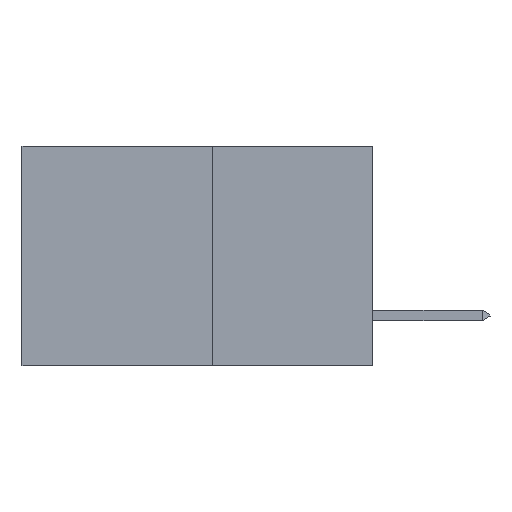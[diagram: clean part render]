
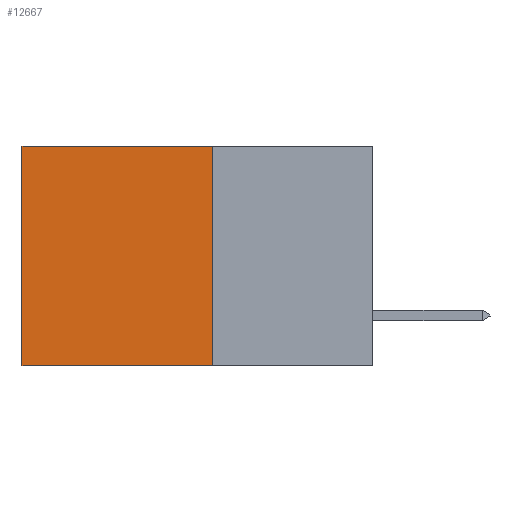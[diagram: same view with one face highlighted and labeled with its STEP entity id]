
A CAD part, left-side view. The second image highlights one B-rep face of the part: STEP entity #12667.
In plain terms, the highlighted planar face has unit normal (-1, 0, 0).
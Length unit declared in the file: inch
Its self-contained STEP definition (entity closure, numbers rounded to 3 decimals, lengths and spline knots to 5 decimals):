
#246 = CARTESIAN_POINT ( 'NONE',  ( 0.277, 0.27, -0.37 ) ) ;
#333 = DIRECTION ( 'NONE',  ( 0., 0., -1. ) ) ;
#2335 = VECTOR ( 'NONE', #3183, 39.37008 ) ;
#2690 = PLANE ( 'NONE',  #11968 ) ;
#3013 = DIRECTION ( 'NONE',  ( 0., 0., -1. ) ) ;
#3183 = DIRECTION ( 'NONE',  ( 0., 1., 0. ) ) ;
#4940 = VECTOR ( 'NONE', #3013, 39.37008 ) ;
#5059 = CARTESIAN_POINT ( 'NONE',  ( 0.277, 0.59, 0. ) ) ;
#5166 = CARTESIAN_POINT ( 'NONE',  ( 0.277, 0.27, 0. ) ) ;
#5239 = EDGE_CURVE ( 'NONE', #13821, #8500, #7722, .T. ) ;
#5249 = FACE_OUTER_BOUND ( 'NONE', #13755, .T. ) ;
#5419 = VECTOR ( 'NONE', #5598, 39.37008 ) ;
#5556 = ORIENTED_EDGE ( 'NONE', *, *, #8982, .F. ) ;
#5598 = DIRECTION ( 'NONE',  ( 0., 0., -1. ) ) ;
#6046 = CARTESIAN_POINT ( 'NONE',  ( 0.277, 0.59, -0.37 ) ) ;
#6131 = LINE ( 'NONE', #5166, #8422 ) ;
#6287 = EDGE_CURVE ( 'NONE', #10686, #8500, #14189, .T. ) ;
#7295 = DIRECTION ( 'NONE',  ( 1., 0., 0. ) ) ;
#7646 = VERTEX_POINT ( 'NONE', #9174 ) ;
#7713 = ORIENTED_EDGE ( 'NONE', *, *, #5239, .F. ) ;
#7722 = LINE ( 'NONE', #246, #2335 ) ;
#8309 = LINE ( 'NONE', #12003, #4940 ) ;
#8422 = VECTOR ( 'NONE', #10748, 39.37008 ) ;
#8500 = VERTEX_POINT ( 'NONE', #9016 ) ;
#8982 = EDGE_CURVE ( 'NONE', #7646, #13821, #8309, .T. ) ;
#9016 = CARTESIAN_POINT ( 'NONE',  ( 0.277, 0.59, -0.37 ) ) ;
#9174 = CARTESIAN_POINT ( 'NONE',  ( 0.277, 0.27, 0. ) ) ;
#10449 = ORIENTED_EDGE ( 'NONE', *, *, #12419, .T. ) ;
#10514 = CARTESIAN_POINT ( 'NONE',  ( 0.277, 0.27, -0.37 ) ) ;
#10686 = VERTEX_POINT ( 'NONE', #5059 ) ;
#10748 = DIRECTION ( 'NONE',  ( 0., 1., 0. ) ) ;
#11238 = ORIENTED_EDGE ( 'NONE', *, *, #6287, .T. ) ;
#11661 = CARTESIAN_POINT ( 'NONE',  ( 0.277, 0.27, -0.37 ) ) ;
#11968 = AXIS2_PLACEMENT_3D ( 'NONE', #11661, #7295, #333 ) ;
#12003 = CARTESIAN_POINT ( 'NONE',  ( 0.277, 0.27, -0.37 ) ) ;
#12419 = EDGE_CURVE ( 'NONE', #7646, #10686, #6131, .T. ) ;
#12667 = ADVANCED_FACE ( 'NONE', ( #5249 ), #2690, .F. ) ;
#13755 = EDGE_LOOP ( 'NONE', ( #11238, #7713, #5556, #10449 ) ) ;
#13821 = VERTEX_POINT ( 'NONE', #10514 ) ;
#14189 = LINE ( 'NONE', #6046, #5419 ) ;
